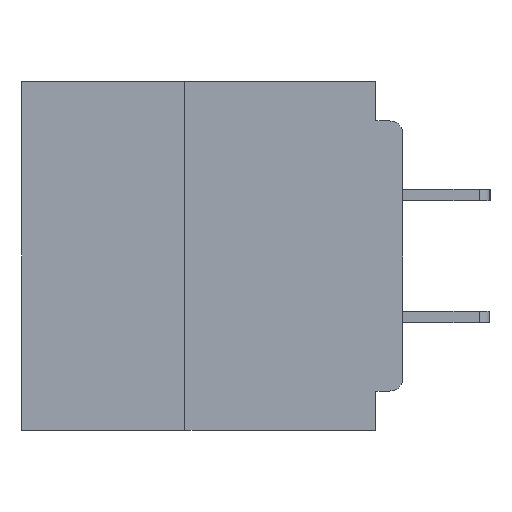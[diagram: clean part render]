
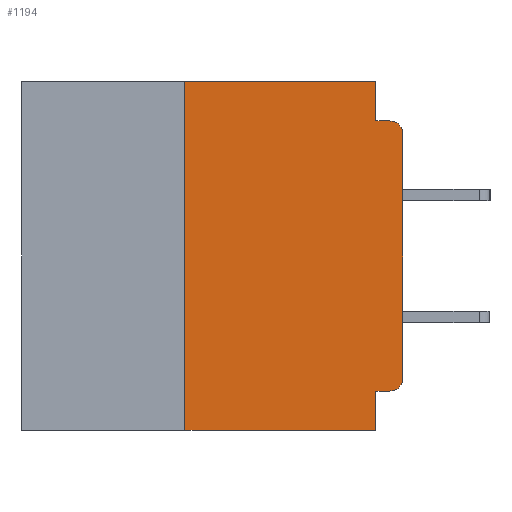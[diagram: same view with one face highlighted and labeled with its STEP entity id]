
A CAD part, left-side view. The second image highlights one B-rep face of the part: STEP entity #1194.
In plain terms, the highlighted planar face has unit normal (-1, 0, 0).
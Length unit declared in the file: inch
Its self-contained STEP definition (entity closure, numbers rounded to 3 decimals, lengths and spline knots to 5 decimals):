
#1194 = ADVANCED_FACE ( 'NONE', ( #33016 ), #13033, .F. ) ;
#2349 = DIRECTION ( 'NONE',  ( 0., 1., 0. ) ) ;
#3129 = VECTOR ( 'NONE', #35397, 39.37008 ) ;
#4017 = VECTOR ( 'NONE', #23033, 39.37008 ) ;
#4332 = CARTESIAN_POINT ( 'NONE',  ( 0., 0., -0.045 ) ) ;
#4370 = ORIENTED_EDGE ( 'NONE', *, *, #5392, .F. ) ;
#5392 = EDGE_CURVE ( 'NONE', #48022, #39834, #35428, .T. ) ;
#6026 = DIRECTION ( 'NONE',  ( 0., 0., -1. ) ) ;
#6819 = DIRECTION ( 'NONE',  ( 0., -1., 0. ) ) ;
#7120 = EDGE_CURVE ( 'NONE', #33023, #36650, #35193, .T. ) ;
#7974 = CARTESIAN_POINT ( 'NONE',  ( 0., 0.031, 0. ) ) ;
#10395 = VERTEX_POINT ( 'NONE', #17330 ) ;
#11123 = ORIENTED_EDGE ( 'NONE', *, *, #31608, .F. ) ;
#11351 = EDGE_CURVE ( 'NONE', #10395, #20839, #29861, .T. ) ;
#11908 = CARTESIAN_POINT ( 'NONE',  ( 0., 0.25, 0. ) ) ;
#12062 = VECTOR ( 'NONE', #2349, 39.37008 ) ;
#12369 = DIRECTION ( 'NONE',  ( 0., 0., 1. ) ) ;
#13033 = PLANE ( 'NONE',  #64695 ) ;
#14148 = ORIENTED_EDGE ( 'NONE', *, *, #7120, .F. ) ;
#14193 = ORIENTED_EDGE ( 'NONE', *, *, #32092, .F. ) ;
#14835 = CARTESIAN_POINT ( 'NONE',  ( 0., 0.031, 0. ) ) ;
#16154 = ORIENTED_EDGE ( 'NONE', *, *, #40431, .T. ) ;
#17330 = CARTESIAN_POINT ( 'NONE',  ( 0., 0.25, -0.4 ) ) ;
#17404 = LINE ( 'NONE', #52979, #4017 ) ;
#17529 = ORIENTED_EDGE ( 'NONE', *, *, #48828, .T. ) ;
#18095 = DIRECTION ( 'NONE',  ( 0., 0., -1. ) ) ;
#19270 = CIRCLE ( 'NONE', #30752, 0.015 ) ;
#19448 = CIRCLE ( 'NONE', #47577, 0.015 ) ;
#20839 = VERTEX_POINT ( 'NONE', #32597 ) ;
#22068 = EDGE_CURVE ( 'NONE', #10395, #48022, #17404, .T. ) ;
#23033 = DIRECTION ( 'NONE',  ( 0., 0., 1. ) ) ;
#24182 = VERTEX_POINT ( 'NONE', #57551 ) ;
#26971 = LINE ( 'NONE', #27612, #12062 ) ;
#27612 = CARTESIAN_POINT ( 'NONE',  ( 0., 0., -0.355 ) ) ;
#28684 = DIRECTION ( 'NONE',  ( -1., 0., 0. ) ) ;
#29684 = CARTESIAN_POINT ( 'NONE',  ( 0., 0.015, -0.34 ) ) ;
#29861 = LINE ( 'NONE', #50225, #3129 ) ;
#30752 = AXIS2_PLACEMENT_3D ( 'NONE', #58618, #28684, #63651 ) ;
#31150 = CARTESIAN_POINT ( 'NONE',  ( 0., 0.031, -0.355 ) ) ;
#31608 = EDGE_CURVE ( 'NONE', #54580, #43335, #26971, .T. ) ;
#31830 = CARTESIAN_POINT ( 'NONE',  ( 0., 0.437, 0. ) ) ;
#32016 = ORIENTED_EDGE ( 'NONE', *, *, #56612, .F. ) ;
#32092 = EDGE_CURVE ( 'NONE', #43335, #20839, #61410, .T. ) ;
#32597 = CARTESIAN_POINT ( 'NONE',  ( 0., 0.031, -0.4 ) ) ;
#33016 = FACE_OUTER_BOUND ( 'NONE', #61008, .T. ) ;
#33023 = VERTEX_POINT ( 'NONE', #53613 ) ;
#34680 = DIRECTION ( 'NONE',  ( 0., 0., -1. ) ) ;
#35193 = LINE ( 'NONE', #4332, #63351 ) ;
#35397 = DIRECTION ( 'NONE',  ( 0., -1., 0. ) ) ;
#35428 = LINE ( 'NONE', #31830, #60446 ) ;
#36150 = VERTEX_POINT ( 'NONE', #52195 ) ;
#36650 = VERTEX_POINT ( 'NONE', #51914 ) ;
#39375 = DIRECTION ( 'NONE',  ( 0., -1., 0. ) ) ;
#39834 = VERTEX_POINT ( 'NONE', #14835 ) ;
#40431 = EDGE_CURVE ( 'NONE', #54580, #24182, #19448, .T. ) ;
#41516 = VECTOR ( 'NONE', #43231, 39.37008 ) ;
#42347 = CARTESIAN_POINT ( 'NONE',  ( 0., 0., 0. ) ) ;
#43231 = DIRECTION ( 'NONE',  ( 0., 0., -1. ) ) ;
#43335 = VERTEX_POINT ( 'NONE', #31150 ) ;
#46105 = CARTESIAN_POINT ( 'NONE',  ( 0., 0.031, -0.4 ) ) ;
#47577 = AXIS2_PLACEMENT_3D ( 'NONE', #29684, #64636, #34680 ) ;
#47820 = CARTESIAN_POINT ( 'NONE',  ( 0., 0.437, 0. ) ) ;
#48022 = VERTEX_POINT ( 'NONE', #11908 ) ;
#48030 = DIRECTION ( 'NONE',  ( 1., 0., 0. ) ) ;
#48828 = EDGE_CURVE ( 'NONE', #36150, #36650, #19270, .T. ) ;
#48929 = VECTOR ( 'NONE', #12369, 39.37008 ) ;
#50225 = CARTESIAN_POINT ( 'NONE',  ( 0., 0.437, -0.4 ) ) ;
#51914 = CARTESIAN_POINT ( 'NONE',  ( 0., 0.015, -0.045 ) ) ;
#52195 = CARTESIAN_POINT ( 'NONE',  ( 0., 0., -0.06 ) ) ;
#52979 = CARTESIAN_POINT ( 'NONE',  ( 0., 0.25, -0.4 ) ) ;
#53613 = CARTESIAN_POINT ( 'NONE',  ( 0., 0.031, -0.045 ) ) ;
#54580 = VERTEX_POINT ( 'NONE', #61921 ) ;
#55971 = ORIENTED_EDGE ( 'NONE', *, *, #63585, .T. ) ;
#56386 = LINE ( 'NONE', #7974, #41516 ) ;
#56612 = EDGE_CURVE ( 'NONE', #39834, #33023, #56386, .T. ) ;
#56815 = ORIENTED_EDGE ( 'NONE', *, *, #22068, .F. ) ;
#57551 = CARTESIAN_POINT ( 'NONE',  ( 0., 0., -0.34 ) ) ;
#58618 = CARTESIAN_POINT ( 'NONE',  ( 0., 0.015, -0.06 ) ) ;
#59827 = VECTOR ( 'NONE', #6026, 39.37008 ) ;
#60008 = ORIENTED_EDGE ( 'NONE', *, *, #11351, .T. ) ;
#60446 = VECTOR ( 'NONE', #6819, 39.37008 ) ;
#60693 = LINE ( 'NONE', #42347, #48929 ) ;
#61008 = EDGE_LOOP ( 'NONE', ( #55971, #17529, #14148, #32016, #4370, #56815, #60008, #14193, #11123, #16154 ) ) ;
#61410 = LINE ( 'NONE', #46105, #59827 ) ;
#61921 = CARTESIAN_POINT ( 'NONE',  ( 0., 0.015, -0.355 ) ) ;
#63351 = VECTOR ( 'NONE', #39375, 39.37008 ) ;
#63585 = EDGE_CURVE ( 'NONE', #24182, #36150, #60693, .T. ) ;
#63651 = DIRECTION ( 'NONE',  ( 0., 0., -1. ) ) ;
#64636 = DIRECTION ( 'NONE',  ( -1., 0., 0. ) ) ;
#64695 = AXIS2_PLACEMENT_3D ( 'NONE', #47820, #48030, #18095 ) ;
